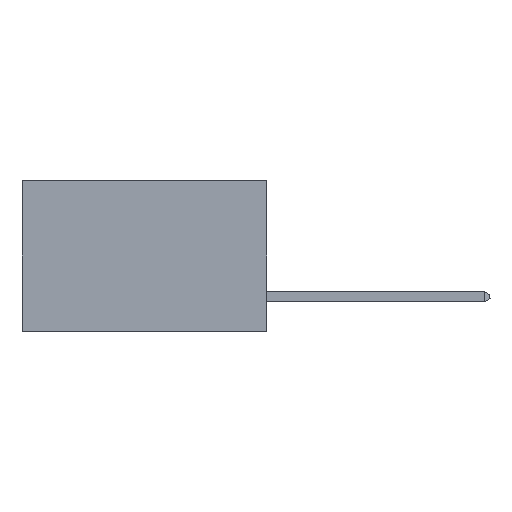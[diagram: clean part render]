
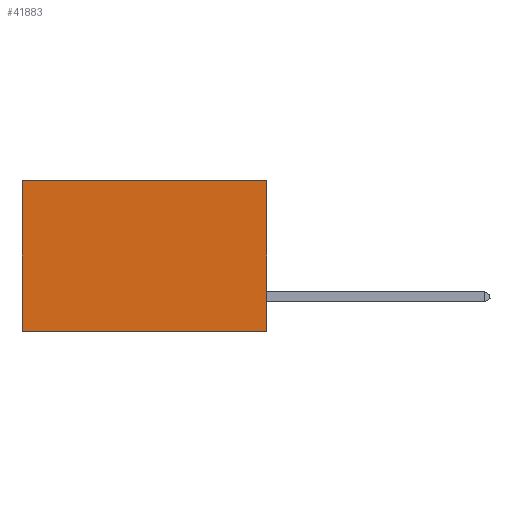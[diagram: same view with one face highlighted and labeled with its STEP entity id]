
A CAD part, left-side view. The second image highlights one B-rep face of the part: STEP entity #41883.
In plain terms, the highlighted planar face has unit normal (-1, 0, 0).
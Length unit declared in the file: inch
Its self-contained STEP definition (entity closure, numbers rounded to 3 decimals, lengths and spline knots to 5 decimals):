
#2143 = VERTEX_POINT ( 'NONE', #29024 ) ;
#2437 = LINE ( 'NONE', #21033, #10330 ) ;
#2818 = DIRECTION ( 'NONE',  ( 1., 0., 0. ) ) ;
#5409 = DIRECTION ( 'NONE',  ( 0., 1., 0. ) ) ;
#5912 = PLANE ( 'NONE',  #34169 ) ;
#7626 = DIRECTION ( 'NONE',  ( 0., 1., 0. ) ) ;
#7689 = ORIENTED_EDGE ( 'NONE', *, *, #10987, .T. ) ;
#10080 = ORIENTED_EDGE ( 'NONE', *, *, #20861, .T. ) ;
#10330 = VECTOR ( 'NONE', #17937, 39.37008 ) ;
#10434 = EDGE_LOOP ( 'NONE', ( #10080, #32658, #39946, #7689 ) ) ;
#10987 = EDGE_CURVE ( 'NONE', #16515, #2143, #31934, .T. ) ;
#12716 = DIRECTION ( 'NONE',  ( 0., 0., -1. ) ) ;
#13525 = CARTESIAN_POINT ( 'NONE',  ( 0.2875, 0.6, -0.37 ) ) ;
#13733 = VERTEX_POINT ( 'NONE', #13525 ) ;
#13969 = EDGE_CURVE ( 'NONE', #16515, #39209, #15856, .T. ) ;
#15017 = FACE_OUTER_BOUND ( 'NONE', #10434, .T. ) ;
#15856 = LINE ( 'NONE', #32450, #42274 ) ;
#16515 = VERTEX_POINT ( 'NONE', #38710 ) ;
#17937 = DIRECTION ( 'NONE',  ( 0., 0., -1. ) ) ;
#19308 = CARTESIAN_POINT ( 'NONE',  ( 0.2875, 0., 0. ) ) ;
#20861 = EDGE_CURVE ( 'NONE', #2143, #13733, #2437, .T. ) ;
#21033 = CARTESIAN_POINT ( 'NONE',  ( 0.2875, 0.6, 0. ) ) ;
#24620 = CARTESIAN_POINT ( 'NONE',  ( 0.2875, 0., -0.37 ) ) ;
#24878 = VECTOR ( 'NONE', #7626, 39.37008 ) ;
#26018 = CARTESIAN_POINT ( 'NONE',  ( 0.2875, 0., 0. ) ) ;
#28739 = VECTOR ( 'NONE', #5409, 39.37008 ) ;
#29024 = CARTESIAN_POINT ( 'NONE',  ( 0.2875, 0.6, 0. ) ) ;
#29234 = CARTESIAN_POINT ( 'NONE',  ( 0.2875, 0., -0.37 ) ) ;
#30547 = EDGE_CURVE ( 'NONE', #39209, #13733, #32870, .T. ) ;
#31934 = LINE ( 'NONE', #19308, #28739 ) ;
#32450 = CARTESIAN_POINT ( 'NONE',  ( 0.2875, 0., 0. ) ) ;
#32658 = ORIENTED_EDGE ( 'NONE', *, *, #30547, .F. ) ;
#32870 = LINE ( 'NONE', #24620, #24878 ) ;
#33353 = DIRECTION ( 'NONE',  ( 0., 0., -1. ) ) ;
#34169 = AXIS2_PLACEMENT_3D ( 'NONE', #26018, #2818, #12716 ) ;
#38710 = CARTESIAN_POINT ( 'NONE',  ( 0.2875, 0., 0. ) ) ;
#39209 = VERTEX_POINT ( 'NONE', #29234 ) ;
#39946 = ORIENTED_EDGE ( 'NONE', *, *, #13969, .F. ) ;
#41883 = ADVANCED_FACE ( 'NONE', ( #15017 ), #5912, .F. ) ;
#42274 = VECTOR ( 'NONE', #33353, 39.37008 ) ;
